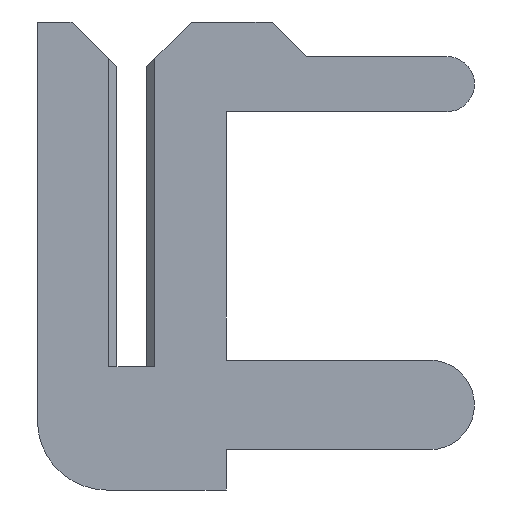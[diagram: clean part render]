
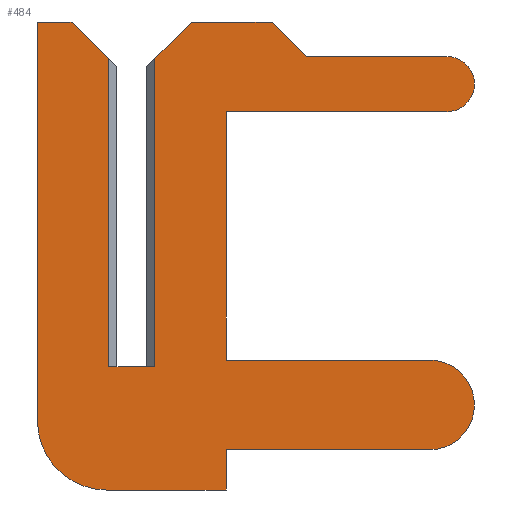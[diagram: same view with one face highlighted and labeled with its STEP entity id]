
A CAD part, left-side view. The second image highlights one B-rep face of the part: STEP entity #484.
In plain terms, the highlighted planar face has unit normal (-1, 0, 0).
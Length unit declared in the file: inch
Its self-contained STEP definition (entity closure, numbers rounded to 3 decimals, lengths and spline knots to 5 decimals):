
#6 = AXIS2_PLACEMENT_3D ( 'NONE', #9, #764, #881 ) ;
#9 = CARTESIAN_POINT ( 'NONE',  ( -0.01, 0.011, -0.0235 ) ) ;
#17 = PLANE ( 'NONE',  #6 ) ;
#26 = DIRECTION ( 'NONE',  ( 0., 0., 1. ) ) ;
#45 = EDGE_CURVE ( 'NONE', #704, #1166, #486, .T. ) ;
#49 = VERTEX_POINT ( 'NONE', #1340 ) ;
#58 = CARTESIAN_POINT ( 'NONE',  ( -0.01, -0.1295, -0.0165 ) ) ;
#70 = VERTEX_POINT ( 'NONE', #152 ) ;
#73 = CARTESIAN_POINT ( 'NONE',  ( -0.01, -0.1295, 0.003 ) ) ;
#74 = CARTESIAN_POINT ( 'NONE',  ( -0.01, -0.041, 0.003 ) ) ;
#77 = EDGE_CURVE ( 'NONE', #104, #301, #1051, .T. ) ;
#94 = CARTESIAN_POINT ( 'NONE',  ( -0.01, -0.076, 0.135 ) ) ;
#97 = DIRECTION ( 'NONE',  ( 0., -0.707, -0.707 ) ) ;
#104 = VERTEX_POINT ( 'NONE', #1364 ) ;
#110 = CARTESIAN_POINT ( 'NONE',  ( -0.01, -0.026, 0.15 ) ) ;
#115 = CARTESIAN_POINT ( 'NONE',  ( -0.01, 0.041, 0.15 ) ) ;
#121 = VECTOR ( 'NONE', #209, 39.37008 ) ;
#137 = CARTESIAN_POINT ( 'NONE',  ( -0.01, -0.137, 0.123 ) ) ;
#152 = CARTESIAN_POINT ( 'NONE',  ( -0.01, 0.01, 0. ) ) ;
#157 = EDGE_CURVE ( 'NONE', #301, #192, #924, .T. ) ;
#162 = CARTESIAN_POINT ( 'NONE',  ( -0.01, -0.1295, 0.003 ) ) ;
#168 = ORIENTED_EDGE ( 'NONE', *, *, #1292, .F. ) ;
#172 = ORIENTED_EDGE ( 'NONE', *, *, #1345, .T. ) ;
#192 = VERTEX_POINT ( 'NONE', #195 ) ;
#195 = CARTESIAN_POINT ( 'NONE',  ( -0.01, -0.061, 0.15 ) ) ;
#197 = VECTOR ( 'NONE', #1092, 39.37008 ) ;
#201 = EDGE_CURVE ( 'NONE', #411, #1233, #1107, .T. ) ;
#203 = CARTESIAN_POINT ( 'NONE',  ( -0.01, -0.041, -0.0535 ) ) ;
#204 = CARTESIAN_POINT ( 'NONE',  ( -0.01, -0.076, 0.135 ) ) ;
#209 = DIRECTION ( 'NONE',  ( 0., 1., 0. ) ) ;
#222 = VERTEX_POINT ( 'NONE', #717 ) ;
#223 = EDGE_CURVE ( 'NONE', #633, #704, #757, .T. ) ;
#229 = LINE ( 'NONE', #667, #197 ) ;
#236 = CARTESIAN_POINT ( 'NONE',  ( -0.01, 0.041, 0.15 ) ) ;
#237 = VERTEX_POINT ( 'NONE', #1378 ) ;
#251 = LINE ( 'NONE', #977, #1052 ) ;
#254 = EDGE_CURVE ( 'NONE', #192, #1047, #419, .T. ) ;
#284 = LINE ( 'NONE', #1241, #121 ) ;
#285 = DIRECTION ( 'NONE',  ( 1., 0., 0. ) ) ;
#288 = LINE ( 'NONE', #1285, #1159 ) ;
#293 = AXIS2_PLACEMENT_3D ( 'NONE', #137, #474, #26 ) ;
#301 = VERTEX_POINT ( 'NONE', #110 ) ;
#303 = DIRECTION ( 'NONE',  ( 0., -0.707, 0.707 ) ) ;
#305 = EDGE_CURVE ( 'NONE', #1047, #1079, #1129, .T. ) ;
#310 = ORIENTED_EDGE ( 'NONE', *, *, #77, .F. ) ;
#322 = EDGE_CURVE ( 'NONE', #1166, #237, #284, .T. ) ;
#324 = ORIENTED_EDGE ( 'NONE', *, *, #254, .F. ) ;
#332 = CARTESIAN_POINT ( 'NONE',  ( -0.01, -0.1295, -0.036 ) ) ;
#358 = DIRECTION ( 'NONE',  ( 0., 1., 0. ) ) ;
#372 = DIRECTION ( 'NONE',  ( 0., -0.707, -0.707 ) ) ;
#373 = VECTOR ( 'NONE', #303, 39.37008 ) ;
#376 = EDGE_CURVE ( 'NONE', #1233, #1303, #1067, .T. ) ;
#389 = AXIS2_PLACEMENT_3D ( 'NONE', #1041, #532, #857 ) ;
#391 = VECTOR ( 'NONE', #1251, 39.37008 ) ;
#398 = VERTEX_POINT ( 'NONE', #1277 ) ;
#406 = CARTESIAN_POINT ( 'NONE',  ( -0.01, -0.01, 0. ) ) ;
#411 = VERTEX_POINT ( 'NONE', #753 ) ;
#419 = LINE ( 'NONE', #94, #893 ) ;
#442 = EDGE_CURVE ( 'NONE', #398, #1122, #499, .T. ) ;
#452 = VECTOR ( 'NONE', #926, 39.37008 ) ;
#455 = CARTESIAN_POINT ( 'NONE',  ( -0.01, -0.041, -0.0535 ) ) ;
#457 = DIRECTION ( 'NONE',  ( 0., 1., 0. ) ) ;
#474 = DIRECTION ( 'NONE',  ( 1., 0., 0. ) ) ;
#480 = AXIS2_PLACEMENT_3D ( 'NONE', #58, #285, #594 ) ;
#484 = ADVANCED_FACE ( 'NONE', ( #1274 ), #17, .T. ) ;
#486 = CIRCLE ( 'NONE', #480, 0.0195 ) ;
#499 = LINE ( 'NONE', #1210, #1246 ) ;
#521 = CARTESIAN_POINT ( 'NONE',  ( -0.01, -0.041, 0.003 ) ) ;
#522 = ORIENTED_EDGE ( 'NONE', *, *, #442, .F. ) ;
#532 = DIRECTION ( 'NONE',  ( 1., 0., 0. ) ) ;
#545 = DIRECTION ( 'NONE',  ( 0., -1., 0. ) ) ;
#579 = CARTESIAN_POINT ( 'NONE',  ( -0.01, -0.0065, 0.1305 ) ) ;
#582 = ORIENTED_EDGE ( 'NONE', *, *, #157, .F. ) ;
#594 = DIRECTION ( 'NONE',  ( 0., 0., 1. ) ) ;
#603 = CARTESIAN_POINT ( 'NONE',  ( -0.01, -0.026, 0.15 ) ) ;
#615 = ORIENTED_EDGE ( 'NONE', *, *, #305, .F. ) ;
#633 = VERTEX_POINT ( 'NONE', #74 ) ;
#643 = ORIENTED_EDGE ( 'NONE', *, *, #1369, .F. ) ;
#667 = CARTESIAN_POINT ( 'NONE',  ( -0.01, 0.026, 0.15 ) ) ;
#683 = EDGE_CURVE ( 'NONE', #70, #723, #1194, .T. ) ;
#700 = VECTOR ( 'NONE', #372, 39.37008 ) ;
#704 = VERTEX_POINT ( 'NONE', #162 ) ;
#705 = ORIENTED_EDGE ( 'NONE', *, *, #45, .F. ) ;
#712 = VECTOR ( 'NONE', #743, 39.37008 ) ;
#717 = CARTESIAN_POINT ( 'NONE',  ( -0.01, 0.01, 0.134 ) ) ;
#723 = VERTEX_POINT ( 'NONE', #406 ) ;
#743 = DIRECTION ( 'NONE',  ( 0., 0., -1. ) ) ;
#747 = DIRECTION ( 'NONE',  ( 0., 0., 1. ) ) ;
#753 = CARTESIAN_POINT ( 'NONE',  ( -0.01, 0.011, -0.0535 ) ) ;
#757 = LINE ( 'NONE', #73, #452 ) ;
#758 = LINE ( 'NONE', #1190, #700 ) ;
#764 = DIRECTION ( 'NONE',  ( -1., 0., 0. ) ) ;
#793 = VECTOR ( 'NONE', #1270, 39.37008 ) ;
#811 = VECTOR ( 'NONE', #545, 39.37008 ) ;
#814 = DIRECTION ( 'NONE',  ( 0., -1., 0. ) ) ;
#839 = EDGE_LOOP ( 'NONE', ( #310, #172, #1045, #1371, #1221, #643, #1155, #882, #913, #1138, #1087, #705, #1180, #1012, #522, #168, #615, #324, #582 ) ) ;
#857 = DIRECTION ( 'NONE',  ( 0., 0., 1. ) ) ;
#859 = CARTESIAN_POINT ( 'NONE',  ( -0.01, -0.041, 0.111 ) ) ;
#875 = CARTESIAN_POINT ( 'NONE',  ( -0.01, 0.041, -0.0235 ) ) ;
#881 = DIRECTION ( 'NONE',  ( 0., 0., 1. ) ) ;
#882 = ORIENTED_EDGE ( 'NONE', *, *, #201, .F. ) ;
#893 = VECTOR ( 'NONE', #97, 39.37008 ) ;
#907 = EDGE_CURVE ( 'NONE', #237, #1219, #1090, .T. ) ;
#909 = VECTOR ( 'NONE', #814, 39.37008 ) ;
#913 = ORIENTED_EDGE ( 'NONE', *, *, #1222, .F. ) ;
#924 = LINE ( 'NONE', #603, #391 ) ;
#926 = DIRECTION ( 'NONE',  ( 0., -1., 0. ) ) ;
#928 = DIRECTION ( 'NONE',  ( 0., 0., -1. ) ) ;
#930 = EDGE_CURVE ( 'NONE', #1122, #633, #1380, .T. ) ;
#959 = CARTESIAN_POINT ( 'NONE',  ( -0.01, -0.137, 0.135 ) ) ;
#969 = LINE ( 'NONE', #1208, #1089 ) ;
#977 = CARTESIAN_POINT ( 'NONE',  ( -0.01, -0.01, 0.15 ) ) ;
#1012 = ORIENTED_EDGE ( 'NONE', *, *, #930, .F. ) ;
#1024 = VECTOR ( 'NONE', #928, 39.37008 ) ;
#1041 = CARTESIAN_POINT ( 'NONE',  ( -0.01, 0.011, -0.0235 ) ) ;
#1045 = ORIENTED_EDGE ( 'NONE', *, *, #683, .F. ) ;
#1047 = VERTEX_POINT ( 'NONE', #204 ) ;
#1051 = LINE ( 'NONE', #579, #373 ) ;
#1052 = VECTOR ( 'NONE', #1320, 39.37008 ) ;
#1067 = LINE ( 'NONE', #115, #793 ) ;
#1079 = VERTEX_POINT ( 'NONE', #1370 ) ;
#1087 = ORIENTED_EDGE ( 'NONE', *, *, #322, .F. ) ;
#1089 = VECTOR ( 'NONE', #457, 39.37008 ) ;
#1090 = LINE ( 'NONE', #203, #1024 ) ;
#1092 = DIRECTION ( 'NONE',  ( 0., -1., 0. ) ) ;
#1107 = CIRCLE ( 'NONE', #389, 0.03 ) ;
#1122 = VERTEX_POINT ( 'NONE', #859 ) ;
#1129 = LINE ( 'NONE', #959, #811 ) ;
#1138 = ORIENTED_EDGE ( 'NONE', *, *, #907, .F. ) ;
#1155 = ORIENTED_EDGE ( 'NONE', *, *, #376, .F. ) ;
#1159 = VECTOR ( 'NONE', #747, 39.37008 ) ;
#1166 = VERTEX_POINT ( 'NONE', #332 ) ;
#1170 = EDGE_CURVE ( 'NONE', #70, #222, #288, .T. ) ;
#1180 = ORIENTED_EDGE ( 'NONE', *, *, #223, .F. ) ;
#1190 = CARTESIAN_POINT ( 'NONE',  ( -0.01, 0.0065, 0.1305 ) ) ;
#1194 = LINE ( 'NONE', #1243, #909 ) ;
#1208 = CARTESIAN_POINT ( 'NONE',  ( -0.01, 0.011, -0.0535 ) ) ;
#1210 = CARTESIAN_POINT ( 'NONE',  ( -0.01, -0.041, 0.111 ) ) ;
#1219 = VERTEX_POINT ( 'NONE', #455 ) ;
#1221 = ORIENTED_EDGE ( 'NONE', *, *, #1264, .F. ) ;
#1222 = EDGE_CURVE ( 'NONE', #1219, #411, #969, .T. ) ;
#1233 = VERTEX_POINT ( 'NONE', #875 ) ;
#1241 = CARTESIAN_POINT ( 'NONE',  ( -0.01, -0.041, -0.036 ) ) ;
#1243 = CARTESIAN_POINT ( 'NONE',  ( -0.01, 0.0065, 0. ) ) ;
#1246 = VECTOR ( 'NONE', #358, 39.37008 ) ;
#1251 = DIRECTION ( 'NONE',  ( 0., -1., 0. ) ) ;
#1264 = EDGE_CURVE ( 'NONE', #49, #222, #758, .T. ) ;
#1270 = DIRECTION ( 'NONE',  ( 0., 0., 1. ) ) ;
#1274 = FACE_OUTER_BOUND ( 'NONE', #839, .T. ) ;
#1277 = CARTESIAN_POINT ( 'NONE',  ( -0.01, -0.137, 0.111 ) ) ;
#1285 = CARTESIAN_POINT ( 'NONE',  ( -0.01, 0.01, -0.0235 ) ) ;
#1292 = EDGE_CURVE ( 'NONE', #1079, #398, #1354, .T. ) ;
#1303 = VERTEX_POINT ( 'NONE', #236 ) ;
#1320 = DIRECTION ( 'NONE',  ( 0., 0., -1. ) ) ;
#1340 = CARTESIAN_POINT ( 'NONE',  ( -0.01, 0.026, 0.15 ) ) ;
#1345 = EDGE_CURVE ( 'NONE', #104, #723, #251, .T. ) ;
#1354 = CIRCLE ( 'NONE', #293, 0.012 ) ;
#1364 = CARTESIAN_POINT ( 'NONE',  ( -0.01, -0.01, 0.134 ) ) ;
#1369 = EDGE_CURVE ( 'NONE', #1303, #49, #229, .T. ) ;
#1370 = CARTESIAN_POINT ( 'NONE',  ( -0.01, -0.137, 0.135 ) ) ;
#1371 = ORIENTED_EDGE ( 'NONE', *, *, #1170, .T. ) ;
#1378 = CARTESIAN_POINT ( 'NONE',  ( -0.01, -0.041, -0.036 ) ) ;
#1380 = LINE ( 'NONE', #521, #712 ) ;
